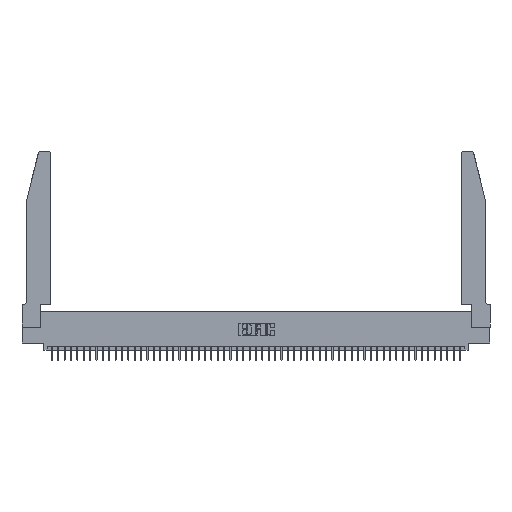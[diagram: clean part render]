
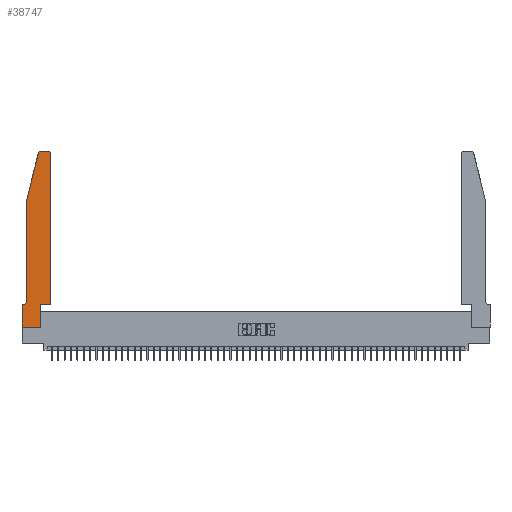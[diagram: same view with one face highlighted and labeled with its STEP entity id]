
A CAD part, top view. The second image highlights one B-rep face of the part: STEP entity #38747.
In plain terms, the highlighted planar face has unit normal (0, 0, 1).
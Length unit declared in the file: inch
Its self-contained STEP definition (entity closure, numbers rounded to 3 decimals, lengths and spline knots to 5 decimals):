
#140 = DIRECTION ( 'NONE',  ( 0., 0., 1. ) ) ;
#540 = VERTEX_POINT ( 'NONE', #9669 ) ;
#561 = VECTOR ( 'NONE', #7367, 39.37008 ) ;
#1160 = CARTESIAN_POINT ( 'NONE',  ( 0.0755, 2., 0.37 ) ) ;
#1298 = CARTESIAN_POINT ( 'NONE',  ( 0.0755, 2., 0.37 ) ) ;
#2625 = DIRECTION ( 'NONE',  ( 1., 0., 0. ) ) ;
#3096 = CARTESIAN_POINT ( 'NONE',  ( 0.0055, 0.35, 0.37 ) ) ;
#3227 = ORIENTED_EDGE ( 'NONE', *, *, #38246, .T. ) ;
#3743 = LINE ( 'NONE', #35326, #25581 ) ;
#3803 = EDGE_CURVE ( 'NONE', #22545, #20997, #50007, .T. ) ;
#3985 = DIRECTION ( 'NONE',  ( 0., 1., 0. ) ) ;
#4368 = DIRECTION ( 'NONE',  ( 1., 0., 0. ) ) ;
#4416 = AXIS2_PLACEMENT_3D ( 'NONE', #32296, #7917, #36401 ) ;
#4642 = LINE ( 'NONE', #1298, #46792 ) ;
#4838 = VERTEX_POINT ( 'NONE', #45186 ) ;
#6075 = DIRECTION ( 'NONE',  ( 0., 0., -1. ) ) ;
#6182 = EDGE_CURVE ( 'NONE', #38124, #22545, #47238, .T. ) ;
#6428 = VERTEX_POINT ( 'NONE', #18189 ) ;
#6703 = VERTEX_POINT ( 'NONE', #20108 ) ;
#6963 = VECTOR ( 'NONE', #46381, 39.37008 ) ;
#7201 = LINE ( 'NONE', #34024, #27660 ) ;
#7367 = DIRECTION ( 'NONE',  ( 0., -1., 0. ) ) ;
#7917 = DIRECTION ( 'NONE',  ( 0., 0., 1. ) ) ;
#7967 = VECTOR ( 'NONE', #3985, 39.37008 ) ;
#8543 = CARTESIAN_POINT ( 'NONE',  ( 0., 0., 0.37 ) ) ;
#9291 = EDGE_CURVE ( 'NONE', #11825, #6703, #49558, .T. ) ;
#9669 = CARTESIAN_POINT ( 'NONE',  ( 0.0755, 2., 0.37 ) ) ;
#11497 = DIRECTION ( 'NONE',  ( 0., 0., 1. ) ) ;
#11586 = ORIENTED_EDGE ( 'NONE', *, *, #9291, .T. ) ;
#11825 = VERTEX_POINT ( 'NONE', #52239 ) ;
#12661 = VECTOR ( 'NONE', #29044, 39.37008 ) ;
#12675 = CARTESIAN_POINT ( 'NONE',  ( 0.2605, 2.75, 0.37 ) ) ;
#13038 = LINE ( 'NONE', #45414, #52469 ) ;
#13166 = ORIENTED_EDGE ( 'NONE', *, *, #37772, .T. ) ;
#14663 = EDGE_CURVE ( 'NONE', #24591, #540, #4642, .T. ) ;
#15443 = CARTESIAN_POINT ( 'NONE',  ( 0., 0., 0.37 ) ) ;
#16163 = EDGE_CURVE ( 'NONE', #6428, #38124, #22478, .T. ) ;
#17899 = CARTESIAN_POINT ( 'NONE',  ( 0.4505, 0.35, 0.37 ) ) ;
#18189 = CARTESIAN_POINT ( 'NONE',  ( 0., 0.35, 0.37 ) ) ;
#18799 = CARTESIAN_POINT ( 'NONE',  ( 0.2865, 0., 0.37 ) ) ;
#19815 = ORIENTED_EDGE ( 'NONE', *, *, #3803, .T. ) ;
#20108 = CARTESIAN_POINT ( 'NONE',  ( 0.4205, 2.75, 0.37 ) ) ;
#20176 = CARTESIAN_POINT ( 'NONE',  ( 0., 0., 0.37 ) ) ;
#20997 = VERTEX_POINT ( 'NONE', #48254 ) ;
#22063 = CIRCLE ( 'NONE', #30329, 0.03 ) ;
#22478 = LINE ( 'NONE', #15443, #561 ) ;
#22545 = VERTEX_POINT ( 'NONE', #18799 ) ;
#22807 = ORIENTED_EDGE ( 'NONE', *, *, #43478, .T. ) ;
#22957 = EDGE_CURVE ( 'NONE', #37733, #11825, #13038, .T. ) ;
#24591 = VERTEX_POINT ( 'NONE', #26854 ) ;
#24883 = ORIENTED_EDGE ( 'NONE', *, *, #16163, .T. ) ;
#25581 = VECTOR ( 'NONE', #2625, 39.37008 ) ;
#26086 = DIRECTION ( 'NONE',  ( -0.239, -0.971, 0. ) ) ;
#26854 = CARTESIAN_POINT ( 'NONE',  ( 0.25487, 2.72718, 0.37 ) ) ;
#26891 = ORIENTED_EDGE ( 'NONE', *, *, #45093, .T. ) ;
#27660 = VECTOR ( 'NONE', #38133, 39.37008 ) ;
#28657 = ORIENTED_EDGE ( 'NONE', *, *, #6182, .T. ) ;
#28698 = VERTEX_POINT ( 'NONE', #3096 ) ;
#28827 = DIRECTION ( 'NONE',  ( 1., 0., 0. ) ) ;
#29044 = DIRECTION ( 'NONE',  ( -1., 0., 0. ) ) ;
#30329 = AXIS2_PLACEMENT_3D ( 'NONE', #35855, #11497, #39958 ) ;
#30509 = CARTESIAN_POINT ( 'NONE',  ( 0.0055, 0.42, 0.37 ) ) ;
#32296 = CARTESIAN_POINT ( 'NONE',  ( 0.4205, 2.72, 0.37 ) ) ;
#32555 = CARTESIAN_POINT ( 'NONE',  ( 0.2865, 0.35, 0.37 ) ) ;
#32714 = CARTESIAN_POINT ( 'NONE',  ( 0., 0.35, 0.37 ) ) ;
#34024 = CARTESIAN_POINT ( 'NONE',  ( 0.0755, 0.35, 0.37 ) ) ;
#34609 = DIRECTION ( 'NONE',  ( -1., 0., 0. ) ) ;
#35326 = CARTESIAN_POINT ( 'NONE',  ( 0.4505, 0.35, 0.37 ) ) ;
#35855 = CARTESIAN_POINT ( 'NONE',  ( 0.284, 2.72, 0.37 ) ) ;
#36380 = VECTOR ( 'NONE', #4368, 39.37008 ) ;
#36401 = DIRECTION ( 'NONE',  ( 1., 0., 0. ) ) ;
#37012 = AXIS2_PLACEMENT_3D ( 'NONE', #30509, #6075, #34609 ) ;
#37219 = DIRECTION ( 'NONE',  ( 0., 1., 0. ) ) ;
#37700 = EDGE_CURVE ( 'NONE', #540, #44606, #51566, .T. ) ;
#37733 = VERTEX_POINT ( 'NONE', #17899 ) ;
#37772 = EDGE_CURVE ( 'NONE', #44606, #28698, #45197, .T. ) ;
#38124 = VERTEX_POINT ( 'NONE', #20176 ) ;
#38133 = DIRECTION ( 'NONE',  ( -1., 0., 0. ) ) ;
#38246 = EDGE_CURVE ( 'NONE', #6703, #4838, #45149, .T. ) ;
#38747 = ADVANCED_FACE ( 'NONE', ( #41252 ), #49094, .T. ) ;
#39473 = AXIS2_PLACEMENT_3D ( 'NONE', #32714, #140, #28827 ) ;
#39958 = DIRECTION ( 'NONE',  ( 1., 0., 0. ) ) ;
#40759 = EDGE_LOOP ( 'NONE', ( #3227, #41587, #44219, #47430, #13166, #22807, #24883, #28657, #19815, #26891, #41479, #11586 ) ) ;
#41252 = FACE_OUTER_BOUND ( 'NONE', #40759, .T. ) ;
#41257 = EDGE_CURVE ( 'NONE', #4838, #24591, #22063, .T. ) ;
#41479 = ORIENTED_EDGE ( 'NONE', *, *, #22957, .T. ) ;
#41587 = ORIENTED_EDGE ( 'NONE', *, *, #41257, .T. ) ;
#43478 = EDGE_CURVE ( 'NONE', #28698, #6428, #7201, .T. ) ;
#44219 = ORIENTED_EDGE ( 'NONE', *, *, #14663, .T. ) ;
#44606 = VERTEX_POINT ( 'NONE', #52750 ) ;
#45093 = EDGE_CURVE ( 'NONE', #20997, #37733, #3743, .T. ) ;
#45149 = LINE ( 'NONE', #12675, #12661 ) ;
#45186 = CARTESIAN_POINT ( 'NONE',  ( 0.284, 2.75, 0.37 ) ) ;
#45197 = CIRCLE ( 'NONE', #37012, 0.07 ) ;
#45414 = CARTESIAN_POINT ( 'NONE',  ( 0.4505, 0.35, 0.37 ) ) ;
#46381 = DIRECTION ( 'NONE',  ( 0., -1., 0. ) ) ;
#46792 = VECTOR ( 'NONE', #26086, 39.37008 ) ;
#47238 = LINE ( 'NONE', #8543, #36380 ) ;
#47430 = ORIENTED_EDGE ( 'NONE', *, *, #37700, .T. ) ;
#48254 = CARTESIAN_POINT ( 'NONE',  ( 0.2865, 0.35, 0.37 ) ) ;
#49094 = PLANE ( 'NONE',  #39473 ) ;
#49558 = CIRCLE ( 'NONE', #4416, 0.03 ) ;
#50007 = LINE ( 'NONE', #32555, #7967 ) ;
#51566 = LINE ( 'NONE', #1160, #6963 ) ;
#52239 = CARTESIAN_POINT ( 'NONE',  ( 0.4505, 2.72, 0.37 ) ) ;
#52469 = VECTOR ( 'NONE', #37219, 39.37008 ) ;
#52750 = CARTESIAN_POINT ( 'NONE',  ( 0.0755, 0.42, 0.37 ) ) ;
